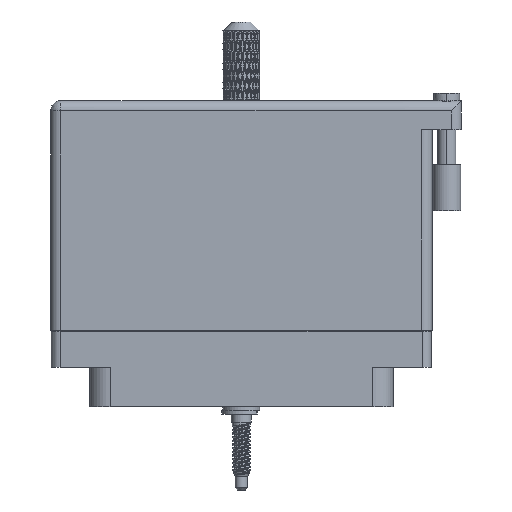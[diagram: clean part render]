
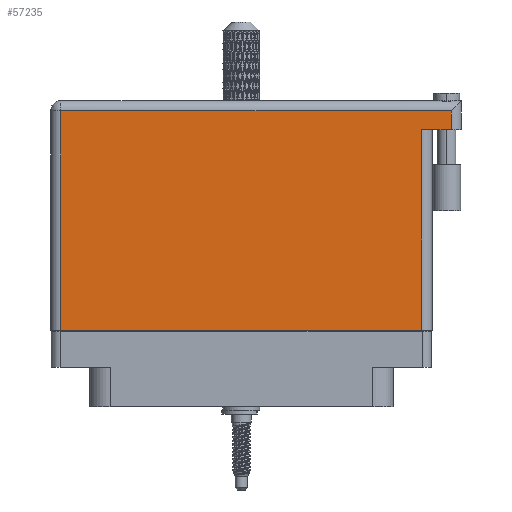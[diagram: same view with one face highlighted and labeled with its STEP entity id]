
A CAD part, front view. The second image highlights one B-rep face of the part: STEP entity #57235.
In plain terms, the highlighted face is planar.
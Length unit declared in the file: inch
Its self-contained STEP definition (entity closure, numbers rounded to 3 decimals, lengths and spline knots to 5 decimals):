
#465 = LINE ( 'NONE', #80306, #53544 ) ;
#634 = LINE ( 'NONE', #41840, #67284 ) ;
#1013 = VECTOR ( 'NONE', #3558, 39.37008 ) ;
#3558 = DIRECTION ( 'NONE',  ( 0., -1., 0. ) ) ;
#8722 = EDGE_LOOP ( 'NONE', ( #92784, #71660, #67819, #28385, #11177, #91369 ) ) ;
#10863 = EDGE_CURVE ( 'NONE', #88230, #86172, #47331, .T. ) ;
#11177 = ORIENTED_EDGE ( 'NONE', *, *, #71582, .T. ) ;
#12805 = LINE ( 'NONE', #24535, #29198 ) ;
#13777 = CARTESIAN_POINT ( 'NONE',  ( 1.23, -0.1, 0.4495 ) ) ;
#14378 = VERTEX_POINT ( 'NONE', #34563 ) ;
#18646 = DIRECTION ( 'NONE',  ( -1., 0., 0. ) ) ;
#21451 = EDGE_CURVE ( 'NONE', #14378, #67455, #82108, .T. ) ;
#24535 = CARTESIAN_POINT ( 'NONE',  ( 1.23, 1.269, 0.4495 ) ) ;
#24646 = EDGE_CURVE ( 'NONE', #81390, #44969, #12805, .T. ) ;
#25914 = CARTESIAN_POINT ( 'NONE',  ( -1.23, 1.396, 0.4495 ) ) ;
#28385 = ORIENTED_EDGE ( 'NONE', *, *, #21451, .T. ) ;
#29198 = VECTOR ( 'NONE', #40850, 39.37008 ) ;
#32193 = CARTESIAN_POINT ( 'NONE',  ( 1.5, 1.269, 0.4495 ) ) ;
#34563 = CARTESIAN_POINT ( 'NONE',  ( 1.43, 1.269, 0.4495 ) ) ;
#40850 = DIRECTION ( 'NONE',  ( 0., 1., 0. ) ) ;
#41840 = CARTESIAN_POINT ( 'NONE',  ( -1.3, -0.1, 0.4495 ) ) ;
#42494 = DIRECTION ( 'NONE',  ( 0., 0., -1. ) ) ;
#44969 = VERTEX_POINT ( 'NONE', #47116 ) ;
#45279 = VECTOR ( 'NONE', #88663, 39.37008 ) ;
#47116 = CARTESIAN_POINT ( 'NONE',  ( 1.23, 1.269, 0.4495 ) ) ;
#47271 = EDGE_CURVE ( 'NONE', #14378, #44969, #100373, .T. ) ;
#47331 = LINE ( 'NONE', #55692, #1013 ) ;
#49963 = VECTOR ( 'NONE', #93103, 39.37008 ) ;
#51715 = DIRECTION ( 'NONE',  ( 1., 0., 0. ) ) ;
#53544 = VECTOR ( 'NONE', #18646, 39.37008 ) ;
#53979 = CARTESIAN_POINT ( 'NONE',  ( 1.43, 1.466, 0.4495 ) ) ;
#55692 = CARTESIAN_POINT ( 'NONE',  ( -1.23, -0.1, 0.4495 ) ) ;
#57235 = ADVANCED_FACE ( 'NONE', ( #77096 ), #58808, .F. ) ;
#58808 = PLANE ( 'NONE',  #85188 ) ;
#67284 = VECTOR ( 'NONE', #51715, 39.37008 ) ;
#67455 = VERTEX_POINT ( 'NONE', #68753 ) ;
#67819 = ORIENTED_EDGE ( 'NONE', *, *, #47271, .F. ) ;
#68753 = CARTESIAN_POINT ( 'NONE',  ( 1.43, 1.396, 0.4495 ) ) ;
#71582 = EDGE_CURVE ( 'NONE', #67455, #88230, #465, .T. ) ;
#71660 = ORIENTED_EDGE ( 'NONE', *, *, #24646, .T. ) ;
#75705 = CARTESIAN_POINT ( 'NONE',  ( -1.23, -0.1, 0.4495 ) ) ;
#77096 = FACE_OUTER_BOUND ( 'NONE', #8722, .T. ) ;
#80306 = CARTESIAN_POINT ( 'NONE',  ( -1.3, 1.396, 0.4495 ) ) ;
#81390 = VERTEX_POINT ( 'NONE', #13777 ) ;
#82108 = LINE ( 'NONE', #53979, #45279 ) ;
#85147 = CARTESIAN_POINT ( 'NONE',  ( -1.3, 1.466, 0.4495 ) ) ;
#85188 = AXIS2_PLACEMENT_3D ( 'NONE', #85147, #42494, #103441 ) ;
#86172 = VERTEX_POINT ( 'NONE', #75705 ) ;
#88230 = VERTEX_POINT ( 'NONE', #25914 ) ;
#88663 = DIRECTION ( 'NONE',  ( 0., 1., 0. ) ) ;
#91369 = ORIENTED_EDGE ( 'NONE', *, *, #10863, .T. ) ;
#92784 = ORIENTED_EDGE ( 'NONE', *, *, #105844, .T. ) ;
#93103 = DIRECTION ( 'NONE',  ( -1., 0., 0. ) ) ;
#100373 = LINE ( 'NONE', #32193, #49963 ) ;
#103441 = DIRECTION ( 'NONE',  ( -1., 0., 0. ) ) ;
#105844 = EDGE_CURVE ( 'NONE', #86172, #81390, #634, .T. ) ;
